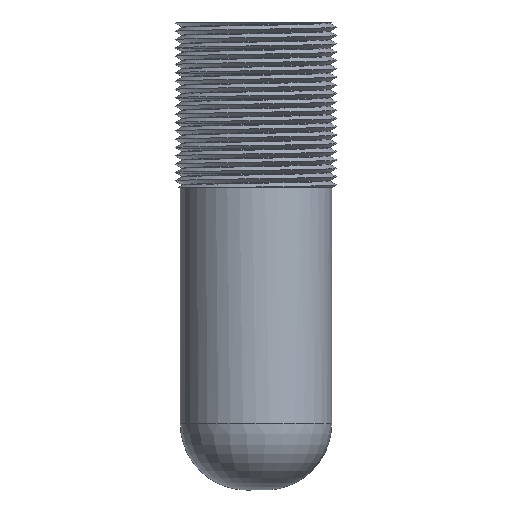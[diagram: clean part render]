
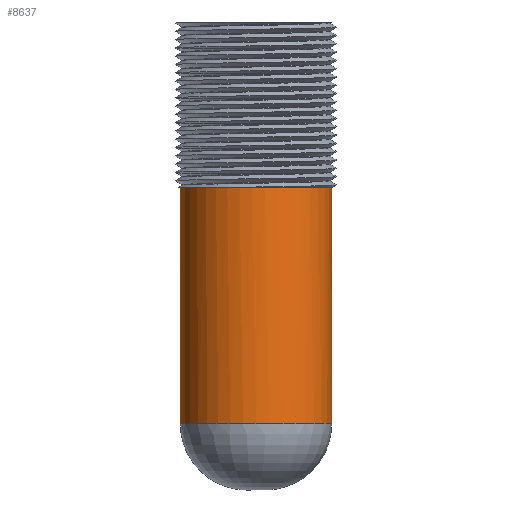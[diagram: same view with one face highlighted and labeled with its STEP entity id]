
A CAD part, front view. The second image highlights one B-rep face of the part: STEP entity #8637.
In plain terms, the highlighted cylindrical face has radius 14.541 mm (diameter 29.083 mm), a full revolution.
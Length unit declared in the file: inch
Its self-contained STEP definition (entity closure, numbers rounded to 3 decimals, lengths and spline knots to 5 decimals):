
#966 = VERTEX_POINT ( 'NONE', #8433 ) ;
#2603 = AXIS2_PLACEMENT_3D ( 'NONE', #27725, #4672, #31585 ) ;
#4672 = DIRECTION ( 'NONE',  ( 0., 0., -1. ) ) ;
#4773 = AXIS2_PLACEMENT_3D ( 'NONE', #10872, #26012, #41606 ) ;
#6751 = ORIENTED_EDGE ( 'NONE', *, *, #34935, .T. ) ;
#8433 = CARTESIAN_POINT ( 'NONE',  ( -0.5725, -0.696, -3.0393 ) ) ;
#8637 = ADVANCED_FACE ( 'NONE', ( #22594, #11145 ), #40587, .T. ) ;
#10551 = EDGE_LOOP ( 'NONE', ( #48338 ) ) ;
#10872 = CARTESIAN_POINT ( 'NONE',  ( 0., -0.696, -1.8956 ) ) ;
#11145 = FACE_OUTER_BOUND ( 'NONE', #28742, .T. ) ;
#11604 = AXIS2_PLACEMENT_3D ( 'NONE', #21031, #47910, #24902 ) ;
#12259 = CIRCLE ( 'NONE', #11604, 0.5725 ) ;
#17588 = AXIS2_PLACEMENT_3D ( 'NONE', #41491, #18488, #45364 ) ;
#18488 = DIRECTION ( 'NONE',  ( 0., 0., 1. ) ) ;
#21031 = CARTESIAN_POINT ( 'NONE',  ( 0., -0.696, -1.25 ) ) ;
#21392 = VERTEX_POINT ( 'NONE', #42985 ) ;
#22594 = FACE_OUTER_BOUND ( 'NONE', #10551, .T. ) ;
#24902 = DIRECTION ( 'NONE',  ( 1., 0., 0. ) ) ;
#26012 = DIRECTION ( 'NONE',  ( 0., 0., -1. ) ) ;
#27725 = CARTESIAN_POINT ( 'NONE',  ( 0., -0.696, -1.25 ) ) ;
#28742 = EDGE_LOOP ( 'NONE', ( #6751, #40710 ) ) ;
#28837 = EDGE_CURVE ( 'NONE', #21392, #31466, #12259, .T. ) ;
#31466 = VERTEX_POINT ( 'NONE', #39123 ) ;
#31585 = DIRECTION ( 'NONE',  ( 1., 0., 0. ) ) ;
#34935 = EDGE_CURVE ( 'NONE', #21392, #31466, #47688, .T. ) ;
#38455 = EDGE_CURVE ( 'NONE', #966, #966, #40453, .T. ) ;
#39123 = CARTESIAN_POINT ( 'NONE',  ( 0.52537, -0.46853, -1.25 ) ) ;
#40453 = CIRCLE ( 'NONE', #17588, 0.5725 ) ;
#40587 = CYLINDRICAL_SURFACE ( 'NONE', #4773, 0.5725 ) ;
#40710 = ORIENTED_EDGE ( 'NONE', *, *, #28837, .F. ) ;
#41491 = CARTESIAN_POINT ( 'NONE',  ( 0., -0.696, -3.0393 ) ) ;
#41606 = DIRECTION ( 'NONE',  ( -1., 0., 0. ) ) ;
#42985 = CARTESIAN_POINT ( 'NONE',  ( -0.38306, -0.27053, -1.25 ) ) ;
#45364 = DIRECTION ( 'NONE',  ( -1., 0., 0. ) ) ;
#47688 = CIRCLE ( 'NONE', #2603, 0.5725 ) ;
#47910 = DIRECTION ( 'NONE',  ( 0., 0., 1. ) ) ;
#48338 = ORIENTED_EDGE ( 'NONE', *, *, #38455, .T. ) ;
